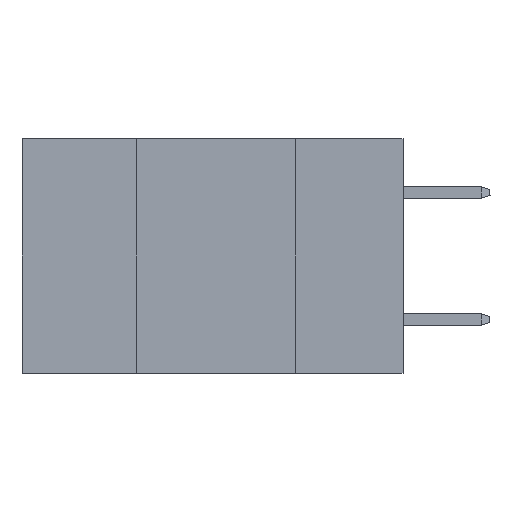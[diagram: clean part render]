
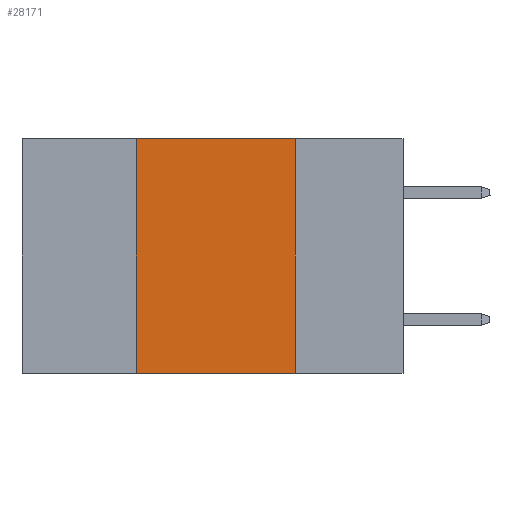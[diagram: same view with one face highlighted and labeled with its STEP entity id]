
A CAD part, left-side view. The second image highlights one B-rep face of the part: STEP entity #28171.
In plain terms, the highlighted planar face has unit normal (-1, 0, 0).
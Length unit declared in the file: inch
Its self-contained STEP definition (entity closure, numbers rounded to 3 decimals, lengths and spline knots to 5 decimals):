
#281 = CARTESIAN_POINT ( 'NONE',  ( 0., 0.42, -0.37 ) ) ;
#2664 = VECTOR ( 'NONE', #23859, 39.37008 ) ;
#2976 = VECTOR ( 'NONE', #32583, 39.37008 ) ;
#3300 = CARTESIAN_POINT ( 'NONE',  ( 0., 0.42, 0. ) ) ;
#5707 = VECTOR ( 'NONE', #34538, 39.37008 ) ;
#6005 = ORIENTED_EDGE ( 'NONE', *, *, #12507, .T. ) ;
#6039 = VERTEX_POINT ( 'NONE', #281 ) ;
#8654 = LINE ( 'NONE', #3300, #2664 ) ;
#9426 = DIRECTION ( 'NONE',  ( 1., 0., 0. ) ) ;
#11848 = LINE ( 'NONE', #29009, #34441 ) ;
#11877 = DIRECTION ( 'NONE',  ( 0., 0., -1. ) ) ;
#11916 = VERTEX_POINT ( 'NONE', #26857 ) ;
#12191 = LINE ( 'NONE', #23452, #2976 ) ;
#12338 = AXIS2_PLACEMENT_3D ( 'NONE', #29411, #9426, #11877 ) ;
#12507 = EDGE_CURVE ( 'NONE', #6039, #33199, #25815, .T. ) ;
#12586 = EDGE_CURVE ( 'NONE', #6039, #13735, #8654, .T. ) ;
#13735 = VERTEX_POINT ( 'NONE', #14893 ) ;
#14893 = CARTESIAN_POINT ( 'NONE',  ( 0., 0.42, 0. ) ) ;
#17573 = DIRECTION ( 'NONE',  ( 0., -1., 0. ) ) ;
#17795 = PLANE ( 'NONE',  #12338 ) ;
#18991 = EDGE_CURVE ( 'NONE', #13735, #11916, #11848, .T. ) ;
#22949 = CARTESIAN_POINT ( 'NONE',  ( 0., 0.6, -0.37 ) ) ;
#23452 = CARTESIAN_POINT ( 'NONE',  ( 0., 0.17, 0. ) ) ;
#23859 = DIRECTION ( 'NONE',  ( 0., 0., 1. ) ) ;
#24381 = ORIENTED_EDGE ( 'NONE', *, *, #12586, .F. ) ;
#25138 = ORIENTED_EDGE ( 'NONE', *, *, #36857, .F. ) ;
#25815 = LINE ( 'NONE', #22949, #5707 ) ;
#26857 = CARTESIAN_POINT ( 'NONE',  ( 0., 0.17, 0. ) ) ;
#28171 = ADVANCED_FACE ( 'NONE', ( #35496 ), #17795, .F. ) ;
#29009 = CARTESIAN_POINT ( 'NONE',  ( 0., 0.6, 0. ) ) ;
#29411 = CARTESIAN_POINT ( 'NONE',  ( 0., 0.6, 0. ) ) ;
#32400 = EDGE_LOOP ( 'NONE', ( #25138, #35059, #24381, #6005 ) ) ;
#32583 = DIRECTION ( 'NONE',  ( 0., 0., -1. ) ) ;
#33199 = VERTEX_POINT ( 'NONE', #36021 ) ;
#34441 = VECTOR ( 'NONE', #17573, 39.37008 ) ;
#34538 = DIRECTION ( 'NONE',  ( 0., -1., 0. ) ) ;
#35059 = ORIENTED_EDGE ( 'NONE', *, *, #18991, .F. ) ;
#35496 = FACE_OUTER_BOUND ( 'NONE', #32400, .T. ) ;
#36021 = CARTESIAN_POINT ( 'NONE',  ( 0., 0.17, -0.37 ) ) ;
#36857 = EDGE_CURVE ( 'NONE', #11916, #33199, #12191, .T. ) ;
